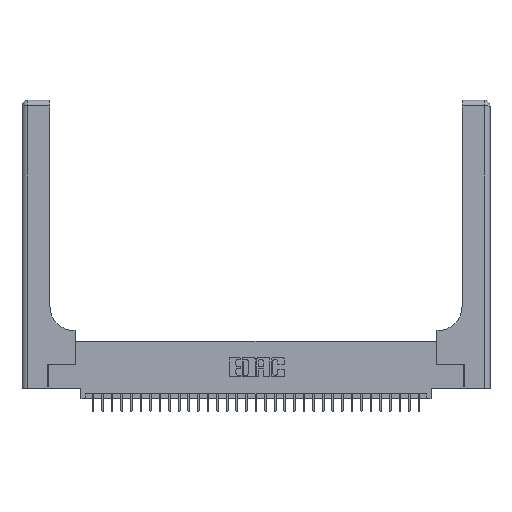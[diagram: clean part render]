
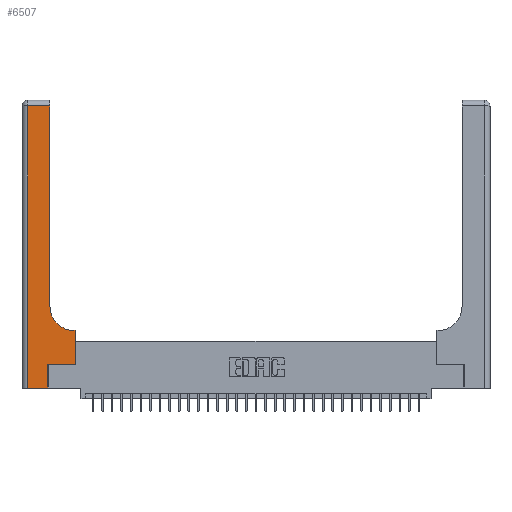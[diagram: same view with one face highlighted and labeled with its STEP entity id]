
A CAD part, top view. The second image highlights one B-rep face of the part: STEP entity #6507.
In plain terms, the highlighted planar face has unit normal (0, 0, 1).
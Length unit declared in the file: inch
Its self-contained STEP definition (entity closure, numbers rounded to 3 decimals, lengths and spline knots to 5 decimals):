
#597 = DIRECTION ( 'NONE',  ( 1., 0., 0. ) ) ;
#612 = EDGE_CURVE ( 'NONE', #24940, #25997, #24233, .T. ) ;
#648 = DIRECTION ( 'NONE',  ( 0., 1., 0. ) ) ;
#1050 = CARTESIAN_POINT ( 'NONE',  ( 0.2915, 0.85, 0.37 ) ) ;
#1483 = CARTESIAN_POINT ( 'NONE',  ( 0.2915, 3., 0.37 ) ) ;
#1693 = ORIENTED_EDGE ( 'NONE', *, *, #10505, .T. ) ;
#1941 = CARTESIAN_POINT ( 'NONE',  ( 0.2915, 0.6, 0.37 ) ) ;
#2292 = DIRECTION ( 'NONE',  ( -1., 0., 0. ) ) ;
#3046 = CARTESIAN_POINT ( 'NONE',  ( 0.5585, 0.25, 0.37 ) ) ;
#3292 = DIRECTION ( 'NONE',  ( 0., 1., 0. ) ) ;
#4015 = ORIENTED_EDGE ( 'NONE', *, *, #21590, .T. ) ;
#5077 = CIRCLE ( 'NONE', #32952, 0.25 ) ;
#5847 = CARTESIAN_POINT ( 'NONE',  ( 0.269, 0., 0.37 ) ) ;
#5950 = LINE ( 'NONE', #31814, #27029 ) ;
#6507 = ADVANCED_FACE ( 'NONE', ( #10007 ), #20450, .F. ) ;
#6553 = LINE ( 'NONE', #6890, #23835 ) ;
#6652 = DIRECTION ( 'NONE',  ( 0., 0., -1. ) ) ;
#6836 = LINE ( 'NONE', #30471, #26002 ) ;
#6890 = CARTESIAN_POINT ( 'NONE',  ( 0., 2.94, 0.37 ) ) ;
#7029 = DIRECTION ( 'NONE',  ( 0., 0., -1. ) ) ;
#7165 = CARTESIAN_POINT ( 'NONE',  ( 0.5415, 0.85, 0.37 ) ) ;
#7591 = CARTESIAN_POINT ( 'NONE',  ( 0.2915, 2.94, 0.37 ) ) ;
#8293 = CARTESIAN_POINT ( 'NONE',  ( 0.06, 0., 0.37 ) ) ;
#8551 = ORIENTED_EDGE ( 'NONE', *, *, #612, .T. ) ;
#10007 = FACE_OUTER_BOUND ( 'NONE', #14638, .T. ) ;
#10505 = EDGE_CURVE ( 'NONE', #28834, #24959, #17226, .T. ) ;
#10563 = VERTEX_POINT ( 'NONE', #20287 ) ;
#11151 = VECTOR ( 'NONE', #597, 39.37008 ) ;
#11812 = ORIENTED_EDGE ( 'NONE', *, *, #14754, .T. ) ;
#12210 = DIRECTION ( 'NONE',  ( -1., 0., 0. ) ) ;
#13212 = ORIENTED_EDGE ( 'NONE', *, *, #20531, .T. ) ;
#13965 = VERTEX_POINT ( 'NONE', #1050 ) ;
#14225 = VERTEX_POINT ( 'NONE', #31167 ) ;
#14490 = DIRECTION ( 'NONE',  ( 0., 1., 0. ) ) ;
#14638 = EDGE_LOOP ( 'NONE', ( #29781, #17501, #4015, #1693, #27937, #8551, #13212, #11812, #29382 ) ) ;
#14754 = EDGE_CURVE ( 'NONE', #14225, #15571, #30874, .T. ) ;
#15571 = VERTEX_POINT ( 'NONE', #22770 ) ;
#16142 = LINE ( 'NONE', #5847, #18992 ) ;
#17226 = LINE ( 'NONE', #27666, #23544 ) ;
#17479 = DIRECTION ( 'NONE',  ( 0., -1., 0. ) ) ;
#17501 = ORIENTED_EDGE ( 'NONE', *, *, #30325, .T. ) ;
#18934 = EDGE_CURVE ( 'NONE', #15571, #13965, #5077, .T. ) ;
#18992 = VECTOR ( 'NONE', #3292, 39.37008 ) ;
#20287 = CARTESIAN_POINT ( 'NONE',  ( 0.06, 2.94, 0.37 ) ) ;
#20450 = PLANE ( 'NONE',  #22305 ) ;
#20531 = EDGE_CURVE ( 'NONE', #25997, #14225, #5950, .T. ) ;
#21590 = EDGE_CURVE ( 'NONE', #10563, #28834, #6836, .T. ) ;
#22305 = AXIS2_PLACEMENT_3D ( 'NONE', #30885, #7029, #32718 ) ;
#22770 = CARTESIAN_POINT ( 'NONE',  ( 0.5415, 0.6, 0.37 ) ) ;
#23544 = VECTOR ( 'NONE', #25443, 39.37008 ) ;
#23562 = VERTEX_POINT ( 'NONE', #7591 ) ;
#23713 = EDGE_CURVE ( 'NONE', #24959, #24940, #16142, .T. ) ;
#23835 = VECTOR ( 'NONE', #12210, 39.37008 ) ;
#24233 = LINE ( 'NONE', #31921, #11151 ) ;
#24940 = VERTEX_POINT ( 'NONE', #28019 ) ;
#24959 = VERTEX_POINT ( 'NONE', #30577 ) ;
#25443 = DIRECTION ( 'NONE',  ( 1., 0., 0. ) ) ;
#25511 = DIRECTION ( 'NONE',  ( 1., 0., 0. ) ) ;
#25997 = VERTEX_POINT ( 'NONE', #3046 ) ;
#26002 = VECTOR ( 'NONE', #17479, 39.37008 ) ;
#26086 = EDGE_CURVE ( 'NONE', #13965, #23562, #30074, .T. ) ;
#27029 = VECTOR ( 'NONE', #648, 39.37008 ) ;
#27666 = CARTESIAN_POINT ( 'NONE',  ( 0., 0., 0.37 ) ) ;
#27937 = ORIENTED_EDGE ( 'NONE', *, *, #23713, .T. ) ;
#28019 = CARTESIAN_POINT ( 'NONE',  ( 0.269, 0.25, 0.37 ) ) ;
#28834 = VERTEX_POINT ( 'NONE', #8293 ) ;
#29382 = ORIENTED_EDGE ( 'NONE', *, *, #18934, .T. ) ;
#29781 = ORIENTED_EDGE ( 'NONE', *, *, #26086, .T. ) ;
#30074 = LINE ( 'NONE', #1483, #32127 ) ;
#30325 = EDGE_CURVE ( 'NONE', #23562, #10563, #6553, .T. ) ;
#30471 = CARTESIAN_POINT ( 'NONE',  ( 0.06, 3., 0.37 ) ) ;
#30577 = CARTESIAN_POINT ( 'NONE',  ( 0.269, 0., 0.37 ) ) ;
#30874 = LINE ( 'NONE', #1941, #33406 ) ;
#30885 = CARTESIAN_POINT ( 'NONE',  ( 0., 3., 0.37 ) ) ;
#31167 = CARTESIAN_POINT ( 'NONE',  ( 0.5585, 0.6, 0.37 ) ) ;
#31814 = CARTESIAN_POINT ( 'NONE',  ( 0.5585, 0.25, 0.37 ) ) ;
#31921 = CARTESIAN_POINT ( 'NONE',  ( 0.269, 0.25, 0.37 ) ) ;
#32127 = VECTOR ( 'NONE', #14490, 39.37008 ) ;
#32718 = DIRECTION ( 'NONE',  ( -1., 0., 0. ) ) ;
#32952 = AXIS2_PLACEMENT_3D ( 'NONE', #7165, #6652, #25511 ) ;
#33406 = VECTOR ( 'NONE', #2292, 39.37008 ) ;
